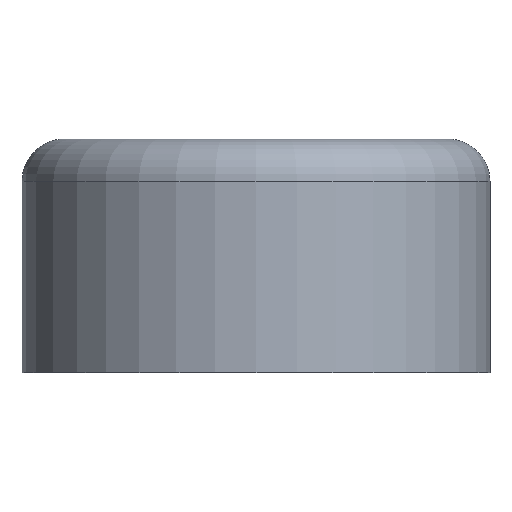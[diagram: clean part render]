
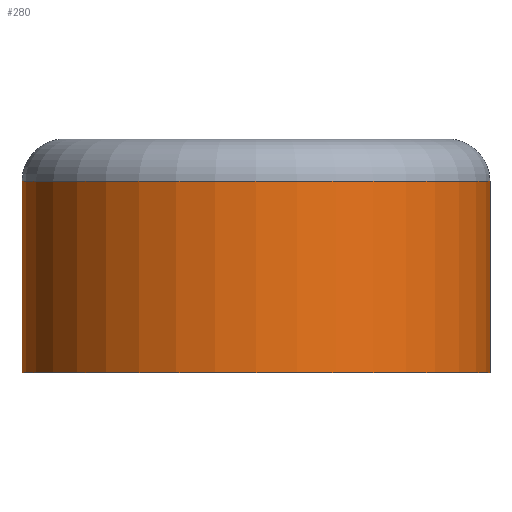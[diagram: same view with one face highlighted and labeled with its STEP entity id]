
A CAD part, front view. The second image highlights one B-rep face of the part: STEP entity #280.
In plain terms, the highlighted cylindrical face has radius 5 mm (diameter 10 mm), a partial arc.
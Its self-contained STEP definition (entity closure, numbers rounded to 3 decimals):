
#9 = VERTEX_POINT ( 'NONE', #243 ) ;
#11 = ORIENTED_EDGE ( 'NONE', *, *, #308, .T. ) ;
#26 = CYLINDRICAL_SURFACE ( 'NONE', #271, 5. ) ;
#28 = DIRECTION ( 'NONE',  ( 0., 0., 1. ) ) ;
#31 = DIRECTION ( 'NONE',  ( 0., 0., -1. ) ) ;
#41 = CIRCLE ( 'NONE', #106, 5. ) ;
#55 = LINE ( 'NONE', #249, #307 ) ;
#57 = CARTESIAN_POINT ( 'NONE',  ( 0., 0., 5. ) ) ;
#73 = VERTEX_POINT ( 'NONE', #197 ) ;
#80 = DIRECTION ( 'NONE',  ( 0., 0., -1. ) ) ;
#84 = CARTESIAN_POINT ( 'NONE',  ( 5., 0., 5. ) ) ;
#87 = ORIENTED_EDGE ( 'NONE', *, *, #315, .T. ) ;
#92 = DIRECTION ( 'NONE',  ( -1., 0., 0. ) ) ;
#104 = AXIS2_PLACEMENT_3D ( 'NONE', #178, #28, #203 ) ;
#106 = AXIS2_PLACEMENT_3D ( 'NONE', #255, #111, #131 ) ;
#111 = DIRECTION ( 'NONE',  ( 0., 0., -1. ) ) ;
#113 = CARTESIAN_POINT ( 'NONE',  ( -5., 0., 0. ) ) ;
#120 = VECTOR ( 'NONE', #31, 1000. ) ;
#122 = EDGE_LOOP ( 'NONE', ( #207, #264, #11, #87 ) ) ;
#131 = DIRECTION ( 'NONE',  ( 1., 0., 0. ) ) ;
#178 = CARTESIAN_POINT ( 'NONE',  ( 0., 0., 0. ) ) ;
#197 = CARTESIAN_POINT ( 'NONE',  ( -5., 0., 4.095 ) ) ;
#203 = DIRECTION ( 'NONE',  ( 1., 0., 0. ) ) ;
#207 = ORIENTED_EDGE ( 'NONE', *, *, #305, .F. ) ;
#220 = CARTESIAN_POINT ( 'NONE',  ( 5., 0., 0. ) ) ;
#226 = CIRCLE ( 'NONE', #104, 5. ) ;
#243 = CARTESIAN_POINT ( 'NONE',  ( 5., 0., 4.095 ) ) ;
#249 = CARTESIAN_POINT ( 'NONE',  ( -5., 0., 5. ) ) ;
#251 = VERTEX_POINT ( 'NONE', #220 ) ;
#255 = CARTESIAN_POINT ( 'NONE',  ( 0., 0., 4.095 ) ) ;
#264 = ORIENTED_EDGE ( 'NONE', *, *, #312, .T. ) ;
#268 = DIRECTION ( 'NONE',  ( 0., 0., -1. ) ) ;
#271 = AXIS2_PLACEMENT_3D ( 'NONE', #57, #80, #92 ) ;
#280 = ADVANCED_FACE ( 'NONE', ( #323 ), #26, .T. ) ;
#294 = VERTEX_POINT ( 'NONE', #113 ) ;
#305 = EDGE_CURVE ( 'NONE', #9, #251, #332, .T. ) ;
#307 = VECTOR ( 'NONE', #268, 1000. ) ;
#308 = EDGE_CURVE ( 'NONE', #73, #294, #55, .T. ) ;
#312 = EDGE_CURVE ( 'NONE', #9, #73, #41, .T. ) ;
#315 = EDGE_CURVE ( 'NONE', #294, #251, #226, .T. ) ;
#323 = FACE_OUTER_BOUND ( 'NONE', #122, .T. ) ;
#332 = LINE ( 'NONE', #84, #120 ) ;
